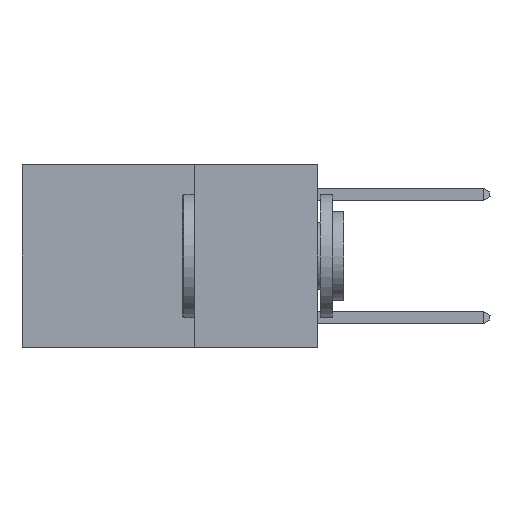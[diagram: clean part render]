
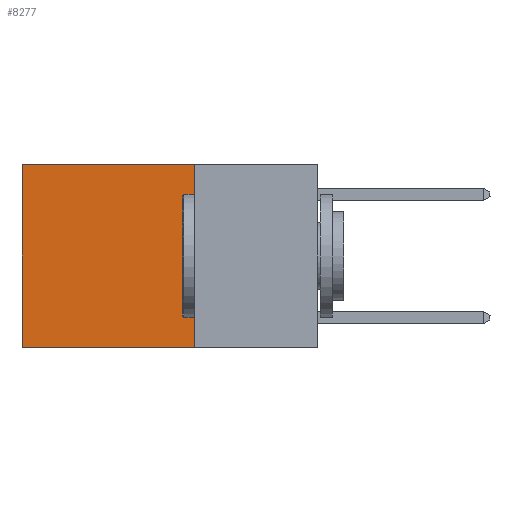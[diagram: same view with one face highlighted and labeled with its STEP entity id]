
A CAD part, left-side view. The second image highlights one B-rep face of the part: STEP entity #8277.
In plain terms, the highlighted planar face has unit normal (-1, 0, 0).
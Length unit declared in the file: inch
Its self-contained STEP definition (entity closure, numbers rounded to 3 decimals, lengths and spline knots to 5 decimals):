
#629 = CARTESIAN_POINT ( 'NONE',  ( 0.2625, 0.25, 0. ) ) ;
#653 = LINE ( 'NONE', #7918, #4762 ) ;
#818 = CARTESIAN_POINT ( 'NONE',  ( 0.2625, 0.25, 0. ) ) ;
#1571 = EDGE_LOOP ( 'NONE', ( #2314, #8499, #7844, #1911 ) ) ;
#1794 = CARTESIAN_POINT ( 'NONE',  ( 0.2625, 0.25, 0. ) ) ;
#1911 = ORIENTED_EDGE ( 'NONE', *, *, #3264, .T. ) ;
#1961 = VECTOR ( 'NONE', #3175, 39.37008 ) ;
#2147 = LINE ( 'NONE', #10885, #12096 ) ;
#2314 = ORIENTED_EDGE ( 'NONE', *, *, #13488, .T. ) ;
#2784 = VERTEX_POINT ( 'NONE', #14074 ) ;
#3175 = DIRECTION ( 'NONE',  ( 0., 0., -1. ) ) ;
#3264 = EDGE_CURVE ( 'NONE', #3702, #2784, #8347, .T. ) ;
#3702 = VERTEX_POINT ( 'NONE', #818 ) ;
#4762 = VECTOR ( 'NONE', #5663, 39.37008 ) ;
#4838 = EDGE_CURVE ( 'NONE', #12179, #5124, #2147, .T. ) ;
#5124 = VERTEX_POINT ( 'NONE', #8149 ) ;
#5609 = EDGE_CURVE ( 'NONE', #3702, #12179, #15531, .T. ) ;
#5663 = DIRECTION ( 'NONE',  ( 0., 0., -1. ) ) ;
#6790 = DIRECTION ( 'NONE',  ( 0., 0., -1. ) ) ;
#7053 = DIRECTION ( 'NONE',  ( 0., 1., 0. ) ) ;
#7055 = DIRECTION ( 'NONE',  ( 0., 1., 0. ) ) ;
#7844 = ORIENTED_EDGE ( 'NONE', *, *, #5609, .F. ) ;
#7918 = CARTESIAN_POINT ( 'NONE',  ( 0.2625, 0.6, 0. ) ) ;
#8004 = PLANE ( 'NONE',  #10112 ) ;
#8043 = VECTOR ( 'NONE', #7053, 39.37008 ) ;
#8065 = CARTESIAN_POINT ( 'NONE',  ( 0.2625, 0.25, -0.37 ) ) ;
#8149 = CARTESIAN_POINT ( 'NONE',  ( 0.2625, 0.6, -0.37 ) ) ;
#8277 = ADVANCED_FACE ( 'NONE', ( #10303 ), #8004, .F. ) ;
#8347 = LINE ( 'NONE', #15743, #8043 ) ;
#8499 = ORIENTED_EDGE ( 'NONE', *, *, #4838, .F. ) ;
#10112 = AXIS2_PLACEMENT_3D ( 'NONE', #1794, #15219, #6790 ) ;
#10303 = FACE_OUTER_BOUND ( 'NONE', #1571, .T. ) ;
#10885 = CARTESIAN_POINT ( 'NONE',  ( 0.2625, 0.25, -0.37 ) ) ;
#12096 = VECTOR ( 'NONE', #7055, 39.37008 ) ;
#12179 = VERTEX_POINT ( 'NONE', #8065 ) ;
#13488 = EDGE_CURVE ( 'NONE', #2784, #5124, #653, .T. ) ;
#14074 = CARTESIAN_POINT ( 'NONE',  ( 0.2625, 0.6, 0. ) ) ;
#15219 = DIRECTION ( 'NONE',  ( 1., 0., 0. ) ) ;
#15531 = LINE ( 'NONE', #629, #1961 ) ;
#15743 = CARTESIAN_POINT ( 'NONE',  ( 0.2625, 0.25, 0. ) ) ;
